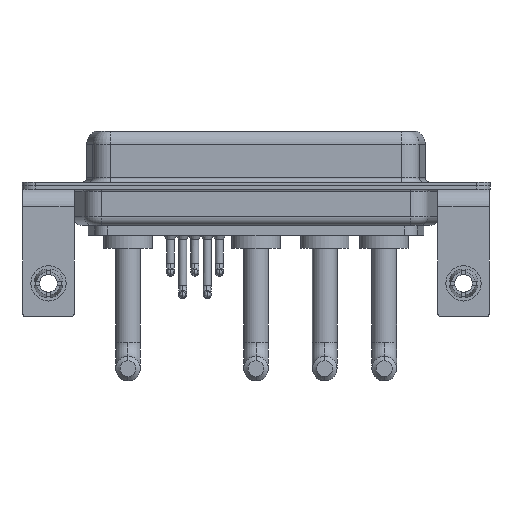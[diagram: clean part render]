
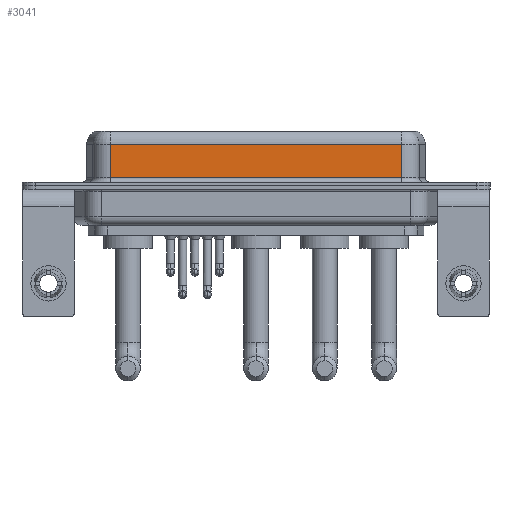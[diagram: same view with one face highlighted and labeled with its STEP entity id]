
A CAD part, front view. The second image highlights one B-rep face of the part: STEP entity #3041.
In plain terms, the highlighted planar face has unit normal (0, -1, 0).
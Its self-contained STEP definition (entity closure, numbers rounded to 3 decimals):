
#672 = CARTESIAN_POINT ( 'NONE',  ( 7.013, -3.95, 6.4 ) ) ;
#845 = VECTOR ( 'NONE', #16514, 1000. ) ;
#2302 = VECTOR ( 'NONE', #5661, 1000. ) ;
#2390 = ORIENTED_EDGE ( 'NONE', *, *, #8502, .T. ) ;
#3041 = ADVANCED_FACE ( 'NONE', ( #11676 ), #7021, .F. ) ;
#3468 = CARTESIAN_POINT ( 'NONE',  ( 7.013, -3.95, 0.9 ) ) ;
#3617 = VECTOR ( 'NONE', #8212, 1000. ) ;
#4234 = DIRECTION ( 'NONE',  ( 0., 1., 0. ) ) ;
#4281 = CARTESIAN_POINT ( 'NONE',  ( 7.013, -3.95, 4.65 ) ) ;
#4318 = EDGE_LOOP ( 'NONE', ( #8693, #2390, #9682, #12842 ) ) ;
#5332 = EDGE_CURVE ( 'NONE', #6000, #14765, #7344, .T. ) ;
#5661 = DIRECTION ( 'NONE',  ( 0., 0., -1. ) ) ;
#6000 = VERTEX_POINT ( 'NONE', #3468 ) ;
#6065 = EDGE_CURVE ( 'NONE', #8585, #6000, #15667, .T. ) ;
#7021 = PLANE ( 'NONE',  #11015 ) ;
#7344 = LINE ( 'NONE', #13393, #14625 ) ;
#7355 = LINE ( 'NONE', #16314, #845 ) ;
#7499 = CARTESIAN_POINT ( 'NONE',  ( 40.037, -3.95, 4.65 ) ) ;
#8212 = DIRECTION ( 'NONE',  ( 0., 0., -1. ) ) ;
#8502 = EDGE_CURVE ( 'NONE', #9599, #8585, #7355, .T. ) ;
#8585 = VERTEX_POINT ( 'NONE', #4281 ) ;
#8693 = ORIENTED_EDGE ( 'NONE', *, *, #10282, .F. ) ;
#9599 = VERTEX_POINT ( 'NONE', #7499 ) ;
#9682 = ORIENTED_EDGE ( 'NONE', *, *, #6065, .T. ) ;
#10022 = CARTESIAN_POINT ( 'NONE',  ( 40.037, -3.95, 6.4 ) ) ;
#10282 = EDGE_CURVE ( 'NONE', #9599, #14765, #14883, .T. ) ;
#10416 = DIRECTION ( 'NONE',  ( 1., 0., 0. ) ) ;
#11015 = AXIS2_PLACEMENT_3D ( 'NONE', #14564, #4234, #19071 ) ;
#11676 = FACE_OUTER_BOUND ( 'NONE', #4318, .T. ) ;
#12842 = ORIENTED_EDGE ( 'NONE', *, *, #5332, .T. ) ;
#13393 = CARTESIAN_POINT ( 'NONE',  ( 40.037, -3.95, 0.9 ) ) ;
#14564 = CARTESIAN_POINT ( 'NONE',  ( 40.037, -3.95, 6.4 ) ) ;
#14625 = VECTOR ( 'NONE', #10416, 1000. ) ;
#14765 = VERTEX_POINT ( 'NONE', #14985 ) ;
#14883 = LINE ( 'NONE', #10022, #2302 ) ;
#14985 = CARTESIAN_POINT ( 'NONE',  ( 40.037, -3.95, 0.9 ) ) ;
#15667 = LINE ( 'NONE', #672, #3617 ) ;
#16314 = CARTESIAN_POINT ( 'NONE',  ( 40.037, -3.95, 4.65 ) ) ;
#16514 = DIRECTION ( 'NONE',  ( -1., 0., 0. ) ) ;
#19071 = DIRECTION ( 'NONE',  ( 0., 0., 1. ) ) ;
